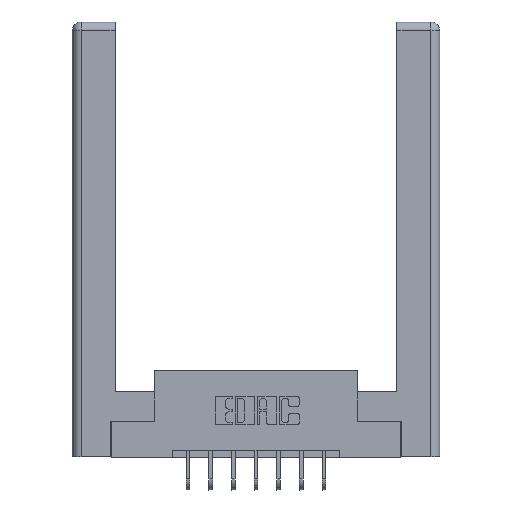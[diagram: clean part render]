
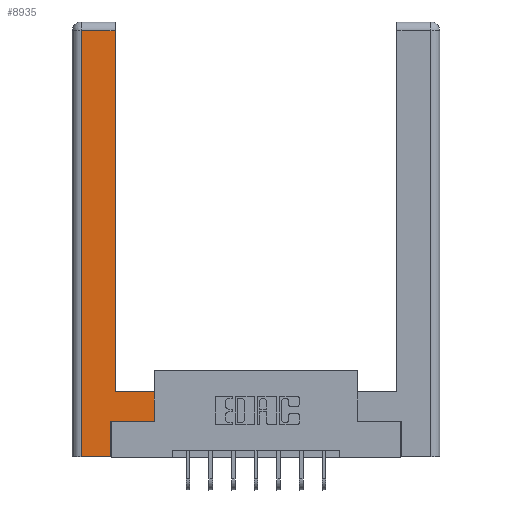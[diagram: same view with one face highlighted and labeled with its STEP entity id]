
A CAD part, top view. The second image highlights one B-rep face of the part: STEP entity #8935.
In plain terms, the highlighted planar face has unit normal (0, 0, 1).
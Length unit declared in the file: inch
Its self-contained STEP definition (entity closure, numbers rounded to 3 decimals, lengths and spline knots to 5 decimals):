
#10 = DIRECTION ( 'NONE',  ( 1., 0., 0. ) ) ;
#297 = ORIENTED_EDGE ( 'NONE', *, *, #9911, .T. ) ;
#790 = PLANE ( 'NONE',  #14244 ) ;
#805 = LINE ( 'NONE', #7778, #11206 ) ;
#880 = CARTESIAN_POINT ( 'NONE',  ( 0.0615, 2.94, 0. ) ) ;
#898 = VECTOR ( 'NONE', #7921, 39.37008 ) ;
#937 = CARTESIAN_POINT ( 'NONE',  ( 0.265, 0.245, 0. ) ) ;
#1045 = LINE ( 'NONE', #9132, #11986 ) ;
#1061 = CARTESIAN_POINT ( 'NONE',  ( 0.565, 0.45, 0. ) ) ;
#1406 = LINE ( 'NONE', #13846, #6642 ) ;
#1425 = EDGE_CURVE ( 'NONE', #12107, #1480, #5748, .T. ) ;
#1480 = VERTEX_POINT ( 'NONE', #937 ) ;
#2154 = ORIENTED_EDGE ( 'NONE', *, *, #1425, .T. ) ;
#2434 = ORIENTED_EDGE ( 'NONE', *, *, #6052, .T. ) ;
#2705 = CARTESIAN_POINT ( 'NONE',  ( 0.265, 0.245, 0. ) ) ;
#3413 = CARTESIAN_POINT ( 'NONE',  ( 0.295, 2.94, 0. ) ) ;
#3641 = ORIENTED_EDGE ( 'NONE', *, *, #10504, .T. ) ;
#4117 = EDGE_CURVE ( 'NONE', #1480, #8349, #805, .T. ) ;
#4629 = VERTEX_POINT ( 'NONE', #3413 ) ;
#4672 = CARTESIAN_POINT ( 'NONE',  ( 0.0615, 0., 0. ) ) ;
#4924 = DIRECTION ( 'NONE',  ( 0., 1., 0. ) ) ;
#5168 = VERTEX_POINT ( 'NONE', #12518 ) ;
#5441 = LINE ( 'NONE', #7871, #898 ) ;
#5590 = VECTOR ( 'NONE', #13827, 39.37008 ) ;
#5666 = ORIENTED_EDGE ( 'NONE', *, *, #8275, .T. ) ;
#5679 = VERTEX_POINT ( 'NONE', #4672 ) ;
#5748 = LINE ( 'NONE', #2705, #12132 ) ;
#6052 = EDGE_CURVE ( 'NONE', #8349, #13753, #6894, .T. ) ;
#6089 = FACE_OUTER_BOUND ( 'NONE', #7402, .T. ) ;
#6252 = DIRECTION ( 'NONE',  ( -1., 0., 0. ) ) ;
#6642 = VECTOR ( 'NONE', #12794, 39.37008 ) ;
#6894 = LINE ( 'NONE', #12006, #10646 ) ;
#6907 = ORIENTED_EDGE ( 'NONE', *, *, #8004, .T. ) ;
#7402 = EDGE_LOOP ( 'NONE', ( #297, #8642, #3641, #6907, #2154, #8335, #2434, #5666 ) ) ;
#7778 = CARTESIAN_POINT ( 'NONE',  ( 0.565, 0.245, 0. ) ) ;
#7871 = CARTESIAN_POINT ( 'NONE',  ( 0.295, 3., 0. ) ) ;
#7921 = DIRECTION ( 'NONE',  ( 0., 1., 0. ) ) ;
#8004 = EDGE_CURVE ( 'NONE', #5679, #12107, #1406, .T. ) ;
#8275 = EDGE_CURVE ( 'NONE', #13753, #5168, #1045, .T. ) ;
#8335 = ORIENTED_EDGE ( 'NONE', *, *, #4117, .T. ) ;
#8349 = VERTEX_POINT ( 'NONE', #12727 ) ;
#8642 = ORIENTED_EDGE ( 'NONE', *, *, #13099, .T. ) ;
#8935 = ADVANCED_FACE ( 'NONE', ( #6089 ), #790, .F. ) ;
#9132 = CARTESIAN_POINT ( 'NONE',  ( 0.295, 0.45, 0. ) ) ;
#9374 = CARTESIAN_POINT ( 'NONE',  ( 0.0615, 0., 0. ) ) ;
#9911 = EDGE_CURVE ( 'NONE', #5168, #4629, #5441, .T. ) ;
#10237 = LINE ( 'NONE', #9374, #5590 ) ;
#10284 = DIRECTION ( 'NONE',  ( -1., 0., 0. ) ) ;
#10504 = EDGE_CURVE ( 'NONE', #14034, #5679, #10237, .T. ) ;
#10612 = DIRECTION ( 'NONE',  ( 0., 0., -1. ) ) ;
#10646 = VECTOR ( 'NONE', #13125, 39.37008 ) ;
#11206 = VECTOR ( 'NONE', #10, 39.37008 ) ;
#11986 = VECTOR ( 'NONE', #10284, 39.37008 ) ;
#11995 = CARTESIAN_POINT ( 'NONE',  ( 0.265, 0., 0. ) ) ;
#12006 = CARTESIAN_POINT ( 'NONE',  ( 0.565, 0.45, 0. ) ) ;
#12107 = VERTEX_POINT ( 'NONE', #11995 ) ;
#12132 = VECTOR ( 'NONE', #4924, 39.37008 ) ;
#12452 = CARTESIAN_POINT ( 'NONE',  ( 0.0615, 2.94, 0. ) ) ;
#12518 = CARTESIAN_POINT ( 'NONE',  ( 0.295, 0.45, 0. ) ) ;
#12573 = LINE ( 'NONE', #880, #13434 ) ;
#12727 = CARTESIAN_POINT ( 'NONE',  ( 0.565, 0.245, 0. ) ) ;
#12794 = DIRECTION ( 'NONE',  ( 1., 0., 0. ) ) ;
#12869 = DIRECTION ( 'NONE',  ( -1., 0., 0. ) ) ;
#13010 = CARTESIAN_POINT ( 'NONE',  ( 0., 0., 0. ) ) ;
#13099 = EDGE_CURVE ( 'NONE', #4629, #14034, #12573, .T. ) ;
#13125 = DIRECTION ( 'NONE',  ( 0., 1., 0. ) ) ;
#13434 = VECTOR ( 'NONE', #6252, 39.37008 ) ;
#13753 = VERTEX_POINT ( 'NONE', #1061 ) ;
#13827 = DIRECTION ( 'NONE',  ( 0., -1., 0. ) ) ;
#13846 = CARTESIAN_POINT ( 'NONE',  ( 0.265, 0., 0. ) ) ;
#14034 = VERTEX_POINT ( 'NONE', #12452 ) ;
#14244 = AXIS2_PLACEMENT_3D ( 'NONE', #13010, #10612, #12869 ) ;
